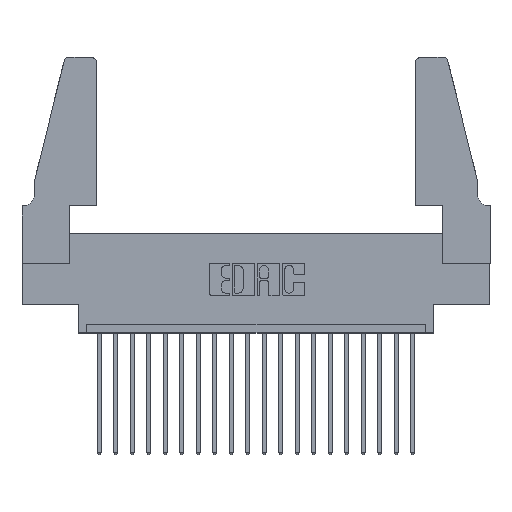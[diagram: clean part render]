
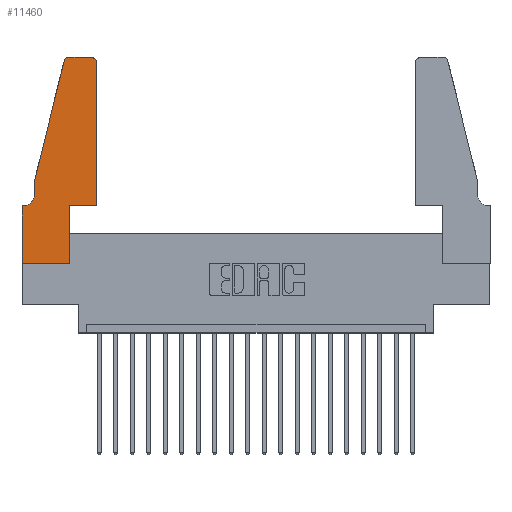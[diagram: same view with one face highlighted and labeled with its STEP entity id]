
A CAD part, top view. The second image highlights one B-rep face of the part: STEP entity #11460.
In plain terms, the highlighted planar face has unit normal (0, 0, 1).
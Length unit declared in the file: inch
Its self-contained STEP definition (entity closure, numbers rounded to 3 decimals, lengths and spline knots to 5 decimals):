
#40 = VECTOR ( 'NONE', #16002, 39.37008 ) ;
#693 = CARTESIAN_POINT ( 'NONE',  ( 0.0755, 0.42, 0.37 ) ) ;
#971 = EDGE_CURVE ( 'NONE', #16119, #5118, #15178, .T. ) ;
#1019 = LINE ( 'NONE', #14497, #40 ) ;
#1148 = LINE ( 'NONE', #11369, #8999 ) ;
#1370 = ORIENTED_EDGE ( 'NONE', *, *, #5718, .T. ) ;
#1587 = VERTEX_POINT ( 'NONE', #19979 ) ;
#1775 = DIRECTION ( 'NONE',  ( -1., 0., 0. ) ) ;
#1926 = CARTESIAN_POINT ( 'NONE',  ( 0.0755, 0.35, 0.37 ) ) ;
#1935 = DIRECTION ( 'NONE',  ( 0., 0., 1. ) ) ;
#2145 = VERTEX_POINT ( 'NONE', #13805 ) ;
#2513 = VERTEX_POINT ( 'NONE', #14662 ) ;
#2538 = LINE ( 'NONE', #6612, #17707 ) ;
#2558 = ORIENTED_EDGE ( 'NONE', *, *, #9012, .T. ) ;
#2629 = LINE ( 'NONE', #1926, #13923 ) ;
#2935 = AXIS2_PLACEMENT_3D ( 'NONE', #10803, #15378, #7592 ) ;
#3073 = CIRCLE ( 'NONE', #2935, 0.07 ) ;
#3234 = CARTESIAN_POINT ( 'NONE',  ( 0.4505, 0.35, 0.37 ) ) ;
#3439 = CARTESIAN_POINT ( 'NONE',  ( 0.0755, 0.5, 0.37 ) ) ;
#3777 = CARTESIAN_POINT ( 'NONE',  ( 0., 0.35, 0.37 ) ) ;
#4461 = AXIS2_PLACEMENT_3D ( 'NONE', #9094, #20082, #13906 ) ;
#4467 = EDGE_CURVE ( 'NONE', #12197, #12922, #5566, .T. ) ;
#4754 = ORIENTED_EDGE ( 'NONE', *, *, #15730, .T. ) ;
#4799 = ORIENTED_EDGE ( 'NONE', *, *, #19624, .T. ) ;
#4890 = EDGE_CURVE ( 'NONE', #1587, #19857, #2629, .T. ) ;
#4952 = DIRECTION ( 'NONE',  ( 0., 0., 1. ) ) ;
#5118 = VERTEX_POINT ( 'NONE', #6097 ) ;
#5311 = VECTOR ( 'NONE', #16612, 39.37008 ) ;
#5566 = LINE ( 'NONE', #7112, #5311 ) ;
#5695 = CIRCLE ( 'NONE', #9659, 0.03 ) ;
#5716 = VERTEX_POINT ( 'NONE', #3439 ) ;
#5718 = EDGE_CURVE ( 'NONE', #8471, #1587, #3073, .T. ) ;
#6097 = CARTESIAN_POINT ( 'NONE',  ( 0.4505, 1.22, 0.37 ) ) ;
#6208 = ORIENTED_EDGE ( 'NONE', *, *, #15956, .T. ) ;
#6215 = LINE ( 'NONE', #20328, #12133 ) ;
#6398 = DIRECTION ( 'NONE',  ( 1., 0., 0. ) ) ;
#6612 = CARTESIAN_POINT ( 'NONE',  ( 0., 0., 0.37 ) ) ;
#6631 = CARTESIAN_POINT ( 'NONE',  ( 0.284, 1.25, 0.37 ) ) ;
#7112 = CARTESIAN_POINT ( 'NONE',  ( 0., 0., 0.37 ) ) ;
#7180 = ORIENTED_EDGE ( 'NONE', *, *, #18742, .T. ) ;
#7559 = EDGE_CURVE ( 'NONE', #2513, #5716, #10352, .T. ) ;
#7592 = DIRECTION ( 'NONE',  ( -1., 0., 0. ) ) ;
#7916 = DIRECTION ( 'NONE',  ( 0., 1., 0. ) ) ;
#8092 = ORIENTED_EDGE ( 'NONE', *, *, #7559, .T. ) ;
#8471 = VERTEX_POINT ( 'NONE', #693 ) ;
#8782 = DIRECTION ( 'NONE',  ( 1., 0., 0. ) ) ;
#8999 = VECTOR ( 'NONE', #10198, 39.37008 ) ;
#9012 = EDGE_CURVE ( 'NONE', #5118, #9034, #5695, .T. ) ;
#9034 = VERTEX_POINT ( 'NONE', #12078 ) ;
#9094 = CARTESIAN_POINT ( 'NONE',  ( 0., 0.35, 0.37 ) ) ;
#9206 = CARTESIAN_POINT ( 'NONE',  ( 0.2865, 0., 0.37 ) ) ;
#9629 = CARTESIAN_POINT ( 'NONE',  ( 0.4505, 0.35, 0.37 ) ) ;
#9659 = AXIS2_PLACEMENT_3D ( 'NONE', #11058, #1935, #8782 ) ;
#10198 = DIRECTION ( 'NONE',  ( 1., 0., 0. ) ) ;
#10352 = LINE ( 'NONE', #18884, #11110 ) ;
#10663 = ORIENTED_EDGE ( 'NONE', *, *, #971, .T. ) ;
#10756 = ORIENTED_EDGE ( 'NONE', *, *, #4890, .T. ) ;
#10803 = CARTESIAN_POINT ( 'NONE',  ( 0.0055, 0.42, 0.37 ) ) ;
#10886 = DIRECTION ( 'NONE',  ( -1., 0., 0. ) ) ;
#11058 = CARTESIAN_POINT ( 'NONE',  ( 0.4205, 1.22, 0.37 ) ) ;
#11110 = VECTOR ( 'NONE', #15592, 39.37008 ) ;
#11369 = CARTESIAN_POINT ( 'NONE',  ( 0.4505, 0.35, 0.37 ) ) ;
#11460 = ADVANCED_FACE ( 'NONE', ( #17626 ), #13774, .T. ) ;
#11614 = CIRCLE ( 'NONE', #13620, 0.03 ) ;
#12078 = CARTESIAN_POINT ( 'NONE',  ( 0.4205, 1.25, 0.37 ) ) ;
#12133 = VECTOR ( 'NONE', #10886, 39.37008 ) ;
#12197 = VERTEX_POINT ( 'NONE', #12526 ) ;
#12526 = CARTESIAN_POINT ( 'NONE',  ( 0., 0., 0.37 ) ) ;
#12922 = VERTEX_POINT ( 'NONE', #9206 ) ;
#13043 = CARTESIAN_POINT ( 'NONE',  ( 0.284, 1.22, 0.37 ) ) ;
#13502 = DIRECTION ( 'NONE',  ( 0., -1., 0. ) ) ;
#13553 = DIRECTION ( 'NONE',  ( 0., 1., 0. ) ) ;
#13620 = AXIS2_PLACEMENT_3D ( 'NONE', #13043, #4952, #6398 ) ;
#13774 = PLANE ( 'NONE',  #4461 ) ;
#13805 = CARTESIAN_POINT ( 'NONE',  ( 0.2865, 0.35, 0.37 ) ) ;
#13906 = DIRECTION ( 'NONE',  ( 1., 0., 0. ) ) ;
#13923 = VECTOR ( 'NONE', #1775, 39.37008 ) ;
#14418 = VECTOR ( 'NONE', #7916, 39.37008 ) ;
#14497 = CARTESIAN_POINT ( 'NONE',  ( 0.0755, 0.5, 0.37 ) ) ;
#14662 = CARTESIAN_POINT ( 'NONE',  ( 0.25487, 1.22718, 0.37 ) ) ;
#14774 = EDGE_CURVE ( 'NONE', #19857, #12197, #2538, .T. ) ;
#15178 = LINE ( 'NONE', #3234, #14418 ) ;
#15378 = DIRECTION ( 'NONE',  ( 0., 0., -1. ) ) ;
#15592 = DIRECTION ( 'NONE',  ( -0.239, -0.971, 0. ) ) ;
#15609 = EDGE_CURVE ( 'NONE', #16649, #2513, #11614, .T. ) ;
#15730 = EDGE_CURVE ( 'NONE', #12922, #2145, #19944, .T. ) ;
#15956 = EDGE_CURVE ( 'NONE', #5716, #8471, #1019, .T. ) ;
#16002 = DIRECTION ( 'NONE',  ( 0., -1., 0. ) ) ;
#16119 = VERTEX_POINT ( 'NONE', #9629 ) ;
#16579 = EDGE_LOOP ( 'NONE', ( #4799, #20239, #8092, #6208, #1370, #10756, #17755, #19005, #4754, #7180, #10663, #2558 ) ) ;
#16612 = DIRECTION ( 'NONE',  ( 1., 0., 0. ) ) ;
#16649 = VERTEX_POINT ( 'NONE', #6631 ) ;
#17232 = VECTOR ( 'NONE', #13553, 39.37008 ) ;
#17626 = FACE_OUTER_BOUND ( 'NONE', #16579, .T. ) ;
#17707 = VECTOR ( 'NONE', #13502, 39.37008 ) ;
#17755 = ORIENTED_EDGE ( 'NONE', *, *, #14774, .T. ) ;
#18742 = EDGE_CURVE ( 'NONE', #2145, #16119, #1148, .T. ) ;
#18884 = CARTESIAN_POINT ( 'NONE',  ( 0.0755, 0.5, 0.37 ) ) ;
#19005 = ORIENTED_EDGE ( 'NONE', *, *, #4467, .T. ) ;
#19624 = EDGE_CURVE ( 'NONE', #9034, #16649, #6215, .T. ) ;
#19793 = CARTESIAN_POINT ( 'NONE',  ( 0.2865, 0.35, 0.37 ) ) ;
#19857 = VERTEX_POINT ( 'NONE', #3777 ) ;
#19944 = LINE ( 'NONE', #19793, #17232 ) ;
#19979 = CARTESIAN_POINT ( 'NONE',  ( 0.0055, 0.35, 0.37 ) ) ;
#20082 = DIRECTION ( 'NONE',  ( 0., 0., 1. ) ) ;
#20239 = ORIENTED_EDGE ( 'NONE', *, *, #15609, .T. ) ;
#20328 = CARTESIAN_POINT ( 'NONE',  ( 0.2605, 1.25, 0.37 ) ) ;
